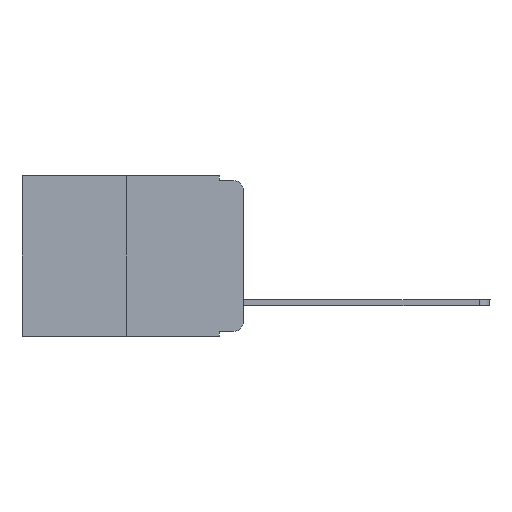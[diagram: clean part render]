
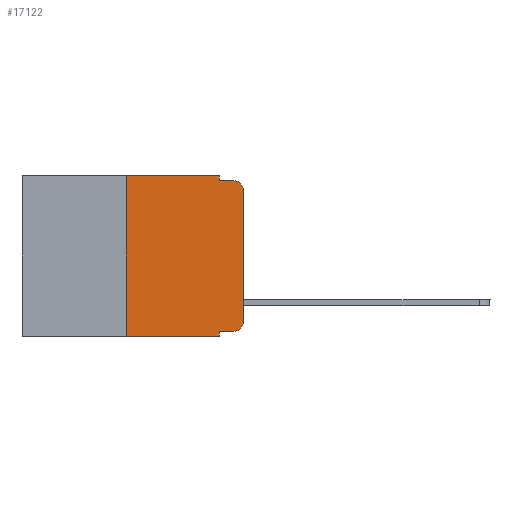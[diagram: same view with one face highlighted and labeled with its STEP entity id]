
A CAD part, left-side view. The second image highlights one B-rep face of the part: STEP entity #17122.
In plain terms, the highlighted planar face has unit normal (-1, 0, 0).
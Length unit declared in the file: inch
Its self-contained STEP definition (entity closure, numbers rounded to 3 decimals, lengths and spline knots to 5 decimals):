
#319 = ORIENTED_EDGE ( 'NONE', *, *, #22728, .T. ) ;
#838 = VERTEX_POINT ( 'NONE', #9206 ) ;
#976 = VECTOR ( 'NONE', #7291, 39.37008 ) ;
#1009 = CIRCLE ( 'NONE', #4164, 0.02 ) ;
#1246 = ORIENTED_EDGE ( 'NONE', *, *, #24611, .F. ) ;
#2183 = EDGE_LOOP ( 'NONE', ( #15927, #22974, #15578, #12651, #18067, #4512, #2763, #1246, #319, #13346 ) ) ;
#2283 = CARTESIAN_POINT ( 'NONE',  ( 0., 0.473, 0. ) ) ;
#2763 = ORIENTED_EDGE ( 'NONE', *, *, #5780, .T. ) ;
#3221 = VERTEX_POINT ( 'NONE', #15970 ) ;
#3833 = VECTOR ( 'NONE', #23038, 39.37008 ) ;
#3883 = LINE ( 'NONE', #24485, #4971 ) ;
#4128 = CARTESIAN_POINT ( 'NONE',  ( 0., 0.051, -0.333 ) ) ;
#4132 = LINE ( 'NONE', #2283, #14596 ) ;
#4164 = AXIS2_PLACEMENT_3D ( 'NONE', #11703, #17450, #19070 ) ;
#4220 = CARTESIAN_POINT ( 'NONE',  ( 0., 0., -0.313 ) ) ;
#4425 = DIRECTION ( 'NONE',  ( 0., 0., 1. ) ) ;
#4512 = ORIENTED_EDGE ( 'NONE', *, *, #20728, .F. ) ;
#4754 = CARTESIAN_POINT ( 'NONE',  ( 0., 0.02, -0.01 ) ) ;
#4801 = LINE ( 'NONE', #23925, #18449 ) ;
#4923 = DIRECTION ( 'NONE',  ( 0., 0., 1. ) ) ;
#4971 = VECTOR ( 'NONE', #13008, 39.37008 ) ;
#5059 = EDGE_CURVE ( 'NONE', #12070, #15085, #22908, .T. ) ;
#5389 = EDGE_CURVE ( 'NONE', #14997, #12070, #9408, .T. ) ;
#5510 = AXIS2_PLACEMENT_3D ( 'NONE', #10198, #12443, #11948 ) ;
#5780 = EDGE_CURVE ( 'NONE', #17181, #838, #3883, .T. ) ;
#5930 = CARTESIAN_POINT ( 'NONE',  ( 0., 0.051, -0.01 ) ) ;
#6495 = DIRECTION ( 'NONE',  ( 0., -1., 0. ) ) ;
#6551 = VERTEX_POINT ( 'NONE', #20399 ) ;
#7042 = EDGE_CURVE ( 'NONE', #3221, #14997, #4132, .T. ) ;
#7291 = DIRECTION ( 'NONE',  ( 0., 0., -1. ) ) ;
#7652 = EDGE_CURVE ( 'NONE', #11552, #15085, #9737, .T. ) ;
#9001 = VECTOR ( 'NONE', #15665, 39.37008 ) ;
#9206 = CARTESIAN_POINT ( 'NONE',  ( 0., 0.051, -0.343 ) ) ;
#9368 = CARTESIAN_POINT ( 'NONE',  ( 0., 0.051, -0.333 ) ) ;
#9408 = LINE ( 'NONE', #17145, #976 ) ;
#9737 = CIRCLE ( 'NONE', #19651, 0.02 ) ;
#9795 = CARTESIAN_POINT ( 'NONE',  ( 0., 0.02, -0.03 ) ) ;
#9991 = LINE ( 'NONE', #4128, #18951 ) ;
#10048 = LINE ( 'NONE', #23047, #11791 ) ;
#10198 = CARTESIAN_POINT ( 'NONE',  ( 0., 0.473, 0. ) ) ;
#11159 = CARTESIAN_POINT ( 'NONE',  ( 0., 0.051, -0.01 ) ) ;
#11552 = VERTEX_POINT ( 'NONE', #22045 ) ;
#11559 = LINE ( 'NONE', #11933, #9001 ) ;
#11703 = CARTESIAN_POINT ( 'NONE',  ( 0., 0.02, -0.313 ) ) ;
#11791 = VECTOR ( 'NONE', #4425, 39.37008 ) ;
#11933 = CARTESIAN_POINT ( 'NONE',  ( 0., 0.051, 0. ) ) ;
#11948 = DIRECTION ( 'NONE',  ( 0., 0., -1. ) ) ;
#12070 = VERTEX_POINT ( 'NONE', #11159 ) ;
#12202 = CARTESIAN_POINT ( 'NONE',  ( 0., 0.25, -0.343 ) ) ;
#12443 = DIRECTION ( 'NONE',  ( 1., 0., 0. ) ) ;
#12587 = EDGE_CURVE ( 'NONE', #6551, #21915, #1009, .T. ) ;
#12651 = ORIENTED_EDGE ( 'NONE', *, *, #5389, .F. ) ;
#13008 = DIRECTION ( 'NONE',  ( 0., -1., 0. ) ) ;
#13283 = DIRECTION ( 'NONE',  ( 0., 0., -1. ) ) ;
#13346 = ORIENTED_EDGE ( 'NONE', *, *, #12587, .T. ) ;
#14596 = VECTOR ( 'NONE', #17500, 39.37008 ) ;
#14997 = VERTEX_POINT ( 'NONE', #18235 ) ;
#15085 = VERTEX_POINT ( 'NONE', #4754 ) ;
#15323 = VERTEX_POINT ( 'NONE', #9368 ) ;
#15578 = ORIENTED_EDGE ( 'NONE', *, *, #5059, .F. ) ;
#15665 = DIRECTION ( 'NONE',  ( 0., 0., -1. ) ) ;
#15927 = ORIENTED_EDGE ( 'NONE', *, *, #24638, .T. ) ;
#15970 = CARTESIAN_POINT ( 'NONE',  ( 0., 0.25, 0. ) ) ;
#17122 = ADVANCED_FACE ( 'NONE', ( #18052 ), #20051, .F. ) ;
#17145 = CARTESIAN_POINT ( 'NONE',  ( 0., 0.051, 0. ) ) ;
#17181 = VERTEX_POINT ( 'NONE', #12202 ) ;
#17450 = DIRECTION ( 'NONE',  ( -1., 0., 0. ) ) ;
#17500 = DIRECTION ( 'NONE',  ( 0., -1., 0. ) ) ;
#18052 = FACE_OUTER_BOUND ( 'NONE', #2183, .T. ) ;
#18067 = ORIENTED_EDGE ( 'NONE', *, *, #7042, .F. ) ;
#18235 = CARTESIAN_POINT ( 'NONE',  ( 0., 0.051, 0. ) ) ;
#18449 = VECTOR ( 'NONE', #4923, 39.37008 ) ;
#18951 = VECTOR ( 'NONE', #6495, 39.37008 ) ;
#19070 = DIRECTION ( 'NONE',  ( 0., 0., -1. ) ) ;
#19651 = AXIS2_PLACEMENT_3D ( 'NONE', #9795, #23032, #13283 ) ;
#20051 = PLANE ( 'NONE',  #5510 ) ;
#20399 = CARTESIAN_POINT ( 'NONE',  ( 0., 0.02, -0.333 ) ) ;
#20728 = EDGE_CURVE ( 'NONE', #17181, #3221, #4801, .T. ) ;
#21915 = VERTEX_POINT ( 'NONE', #4220 ) ;
#22045 = CARTESIAN_POINT ( 'NONE',  ( 0., 0., -0.03 ) ) ;
#22728 = EDGE_CURVE ( 'NONE', #15323, #6551, #9991, .T. ) ;
#22908 = LINE ( 'NONE', #5930, #3833 ) ;
#22974 = ORIENTED_EDGE ( 'NONE', *, *, #7652, .T. ) ;
#23032 = DIRECTION ( 'NONE',  ( -1., 0., 0. ) ) ;
#23038 = DIRECTION ( 'NONE',  ( 0., -1., 0. ) ) ;
#23047 = CARTESIAN_POINT ( 'NONE',  ( 0., 0., 0. ) ) ;
#23925 = CARTESIAN_POINT ( 'NONE',  ( 0., 0.25, 0. ) ) ;
#24485 = CARTESIAN_POINT ( 'NONE',  ( 0., 0.473, -0.343 ) ) ;
#24611 = EDGE_CURVE ( 'NONE', #15323, #838, #11559, .T. ) ;
#24638 = EDGE_CURVE ( 'NONE', #21915, #11552, #10048, .T. ) ;
